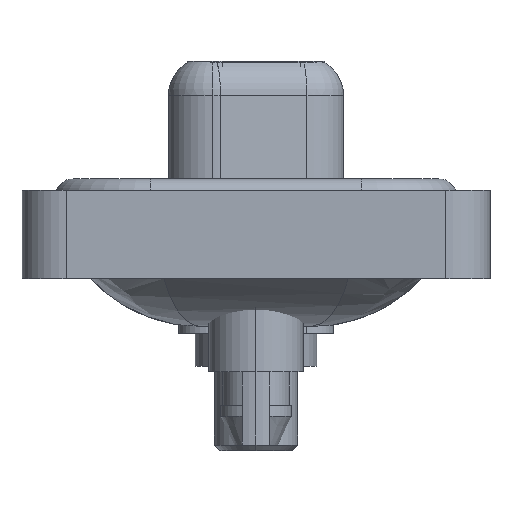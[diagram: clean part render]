
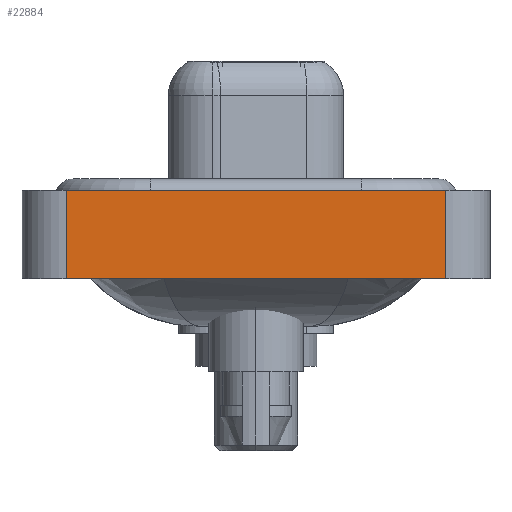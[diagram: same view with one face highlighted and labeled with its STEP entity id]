
A CAD part, left-side view. The second image highlights one B-rep face of the part: STEP entity #22884.
In plain terms, the highlighted planar face has unit normal (-1, 0, 0).
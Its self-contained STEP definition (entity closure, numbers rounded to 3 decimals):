
#425 = AXIS2_PLACEMENT_3D ( 'NONE', #7683, #25551, #11984 ) ;
#740 = CARTESIAN_POINT ( 'NONE',  ( -7.35, 8.55, -3.6 ) ) ;
#2061 = DIRECTION ( 'NONE',  ( 0., -1., 0. ) ) ;
#2236 = DIRECTION ( 'NONE',  ( 0., 0., 1. ) ) ;
#2877 = CARTESIAN_POINT ( 'NONE',  ( -7.35, -8.55, -3.6 ) ) ;
#3184 = CARTESIAN_POINT ( 'NONE',  ( -7.35, 8.55, -3.6 ) ) ;
#3424 = ORIENTED_EDGE ( 'NONE', *, *, #16778, .F. ) ;
#3485 = PLANE ( 'NONE',  #425 ) ;
#3545 = CARTESIAN_POINT ( 'NONE',  ( -7.35, 8.55, 0.4 ) ) ;
#3893 = CARTESIAN_POINT ( 'NONE',  ( -7.35, -8.55, -3.6 ) ) ;
#3908 = LINE ( 'NONE', #20050, #8309 ) ;
#3949 = ORIENTED_EDGE ( 'NONE', *, *, #17640, .T. ) ;
#4216 = LINE ( 'NONE', #740, #9411 ) ;
#5449 = VERTEX_POINT ( 'NONE', #10465 ) ;
#6711 = EDGE_CURVE ( 'NONE', #24442, #5449, #26001, .T. ) ;
#7683 = CARTESIAN_POINT ( 'NONE',  ( -7.35, -8.55, -3.6 ) ) ;
#8309 = VECTOR ( 'NONE', #2061, 1000. ) ;
#8369 = CARTESIAN_POINT ( 'NONE',  ( -7.35, -8.55, -3.6 ) ) ;
#8405 = VERTEX_POINT ( 'NONE', #3545 ) ;
#9411 = VECTOR ( 'NONE', #2236, 1000. ) ;
#10454 = EDGE_CURVE ( 'NONE', #12707, #8405, #4216, .T. ) ;
#10465 = CARTESIAN_POINT ( 'NONE',  ( -7.35, -8.55, 0.4 ) ) ;
#10877 = LINE ( 'NONE', #2877, #21238 ) ;
#11984 = DIRECTION ( 'NONE',  ( 0., 0., 1. ) ) ;
#12707 = VERTEX_POINT ( 'NONE', #3184 ) ;
#14516 = EDGE_LOOP ( 'NONE', ( #25984, #3424, #19577, #3949 ) ) ;
#14670 = DIRECTION ( 'NONE',  ( 0., -1., 0. ) ) ;
#15544 = FACE_OUTER_BOUND ( 'NONE', #14516, .T. ) ;
#16778 = EDGE_CURVE ( 'NONE', #8405, #5449, #3908, .T. ) ;
#17640 = EDGE_CURVE ( 'NONE', #12707, #24442, #10877, .T. ) ;
#18496 = DIRECTION ( 'NONE',  ( 0., 0., 1. ) ) ;
#19577 = ORIENTED_EDGE ( 'NONE', *, *, #10454, .F. ) ;
#20050 = CARTESIAN_POINT ( 'NONE',  ( -7.35, -8.55, 0.4 ) ) ;
#21238 = VECTOR ( 'NONE', #14670, 1000. ) ;
#22884 = ADVANCED_FACE ( 'NONE', ( #15544 ), #3485, .T. ) ;
#24066 = VECTOR ( 'NONE', #18496, 1000. ) ;
#24442 = VERTEX_POINT ( 'NONE', #3893 ) ;
#25551 = DIRECTION ( 'NONE',  ( -1., 0., 0. ) ) ;
#25984 = ORIENTED_EDGE ( 'NONE', *, *, #6711, .T. ) ;
#26001 = LINE ( 'NONE', #8369, #24066 ) ;
